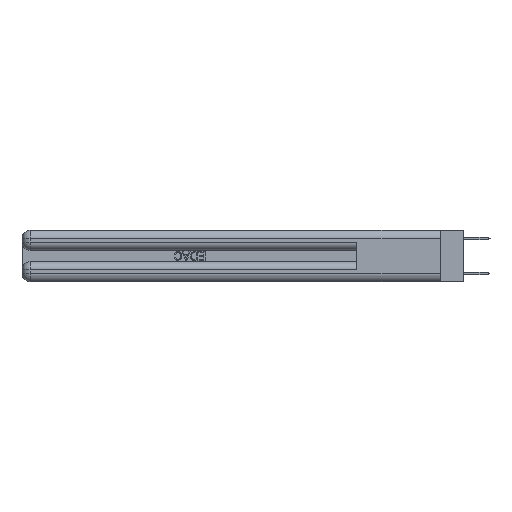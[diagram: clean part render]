
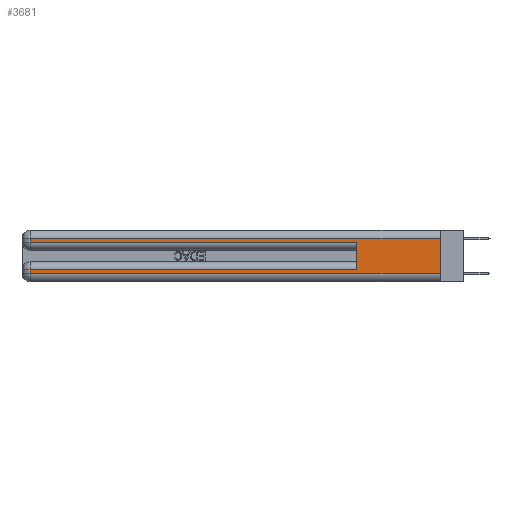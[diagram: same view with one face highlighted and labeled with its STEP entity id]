
A CAD part, left-side view. The second image highlights one B-rep face of the part: STEP entity #3681.
In plain terms, the highlighted planar face has unit normal (-1, 0, 0).
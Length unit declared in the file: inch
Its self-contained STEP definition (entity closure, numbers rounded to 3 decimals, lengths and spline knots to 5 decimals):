
#848 = VECTOR ( 'NONE', #24664, 39.37008 ) ;
#1297 = VERTEX_POINT ( 'NONE', #13700 ) ;
#1699 = DIRECTION ( 'NONE',  ( 0., -1., 0. ) ) ;
#1996 = VERTEX_POINT ( 'NONE', #3003 ) ;
#2020 = CARTESIAN_POINT ( 'NONE',  ( 0., 0., 0.31 ) ) ;
#2105 = ORIENTED_EDGE ( 'NONE', *, *, #17042, .T. ) ;
#2227 = FACE_OUTER_BOUND ( 'NONE', #9442, .T. ) ;
#2357 = LINE ( 'NONE', #11432, #7152 ) ;
#2639 = DIRECTION ( 'NONE',  ( 0., 0., -1. ) ) ;
#2806 = CARTESIAN_POINT ( 'NONE',  ( 0., 2.94, 0.285 ) ) ;
#2885 = CARTESIAN_POINT ( 'NONE',  ( 0., 0., 0.285 ) ) ;
#3003 = CARTESIAN_POINT ( 'NONE',  ( 0., 0.6, 0.085 ) ) ;
#3089 = LINE ( 'NONE', #8901, #11124 ) ;
#3681 = ADVANCED_FACE ( 'NONE', ( #2227 ), #26254, .F. ) ;
#3706 = EDGE_CURVE ( 'NONE', #1996, #14106, #2357, .T. ) ;
#4356 = CARTESIAN_POINT ( 'NONE',  ( 0., 2.94, 0.31 ) ) ;
#4661 = DIRECTION ( 'NONE',  ( 0., 0., -1. ) ) ;
#6040 = LINE ( 'NONE', #21660, #19885 ) ;
#6466 = EDGE_CURVE ( 'NONE', #17110, #20789, #20079, .T. ) ;
#6654 = CARTESIAN_POINT ( 'NONE',  ( 0., 0., 0.37 ) ) ;
#6743 = CARTESIAN_POINT ( 'NONE',  ( 0., 0.6, 0.145 ) ) ;
#7045 = DIRECTION ( 'NONE',  ( 0., 0., -1. ) ) ;
#7152 = VECTOR ( 'NONE', #15279, 39.37008 ) ;
#8901 = CARTESIAN_POINT ( 'NONE',  ( 0., 2.94, 0.37 ) ) ;
#9012 = VERTEX_POINT ( 'NONE', #4356 ) ;
#9410 = EDGE_CURVE ( 'NONE', #26580, #9012, #6040, .T. ) ;
#9442 = EDGE_LOOP ( 'NONE', ( #22428, #20147, #17220, #12533, #23131, #20589, #13946, #2105 ) ) ;
#9989 = VECTOR ( 'NONE', #4661, 39.37008 ) ;
#10642 = LINE ( 'NONE', #6654, #9989 ) ;
#10772 = LINE ( 'NONE', #12498, #20556 ) ;
#10876 = DIRECTION ( 'NONE',  ( 1., 0., 0. ) ) ;
#11124 = VECTOR ( 'NONE', #7045, 39.37008 ) ;
#11432 = CARTESIAN_POINT ( 'NONE',  ( 0., 0., 0.085 ) ) ;
#12150 = VECTOR ( 'NONE', #22633, 39.37008 ) ;
#12498 = CARTESIAN_POINT ( 'NONE',  ( 0., 0., 0.06 ) ) ;
#12533 = ORIENTED_EDGE ( 'NONE', *, *, #6466, .T. ) ;
#13148 = DIRECTION ( 'NONE',  ( 0., 1., 0. ) ) ;
#13305 = EDGE_CURVE ( 'NONE', #26580, #18356, #10642, .T. ) ;
#13700 = CARTESIAN_POINT ( 'NONE',  ( 0., 2.94, 0.06 ) ) ;
#13946 = ORIENTED_EDGE ( 'NONE', *, *, #21067, .T. ) ;
#14106 = VERTEX_POINT ( 'NONE', #22814 ) ;
#15279 = DIRECTION ( 'NONE',  ( 0., 1., 0. ) ) ;
#15874 = CARTESIAN_POINT ( 'NONE',  ( 0., 0., 0.06 ) ) ;
#15970 = LINE ( 'NONE', #6743, #848 ) ;
#17042 = EDGE_CURVE ( 'NONE', #1297, #18356, #10772, .T. ) ;
#17110 = VERTEX_POINT ( 'NONE', #2806 ) ;
#17220 = ORIENTED_EDGE ( 'NONE', *, *, #19306, .T. ) ;
#18356 = VERTEX_POINT ( 'NONE', #15874 ) ;
#19306 = EDGE_CURVE ( 'NONE', #9012, #17110, #3089, .T. ) ;
#19885 = VECTOR ( 'NONE', #13148, 39.37008 ) ;
#19966 = CARTESIAN_POINT ( 'NONE',  ( 0., 2.94, 0.37 ) ) ;
#20079 = LINE ( 'NONE', #2885, #12150 ) ;
#20147 = ORIENTED_EDGE ( 'NONE', *, *, #9410, .T. ) ;
#20248 = DIRECTION ( 'NONE',  ( 0., 0., -1. ) ) ;
#20556 = VECTOR ( 'NONE', #1699, 39.37008 ) ;
#20589 = ORIENTED_EDGE ( 'NONE', *, *, #3706, .T. ) ;
#20789 = VERTEX_POINT ( 'NONE', #22726 ) ;
#21067 = EDGE_CURVE ( 'NONE', #14106, #1297, #24092, .T. ) ;
#21090 = EDGE_CURVE ( 'NONE', #1996, #20789, #15970, .T. ) ;
#21660 = CARTESIAN_POINT ( 'NONE',  ( 0., 0., 0.31 ) ) ;
#21690 = AXIS2_PLACEMENT_3D ( 'NONE', #22088, #10876, #2639 ) ;
#22088 = CARTESIAN_POINT ( 'NONE',  ( 0., 0., 0.37 ) ) ;
#22428 = ORIENTED_EDGE ( 'NONE', *, *, #13305, .F. ) ;
#22633 = DIRECTION ( 'NONE',  ( 0., -1., 0. ) ) ;
#22726 = CARTESIAN_POINT ( 'NONE',  ( 0., 0.6, 0.285 ) ) ;
#22814 = CARTESIAN_POINT ( 'NONE',  ( 0., 2.94, 0.085 ) ) ;
#23131 = ORIENTED_EDGE ( 'NONE', *, *, #21090, .F. ) ;
#24092 = LINE ( 'NONE', #19966, #26724 ) ;
#24664 = DIRECTION ( 'NONE',  ( 0., 0., 1. ) ) ;
#26254 = PLANE ( 'NONE',  #21690 ) ;
#26580 = VERTEX_POINT ( 'NONE', #2020 ) ;
#26724 = VECTOR ( 'NONE', #20248, 39.37008 ) ;
